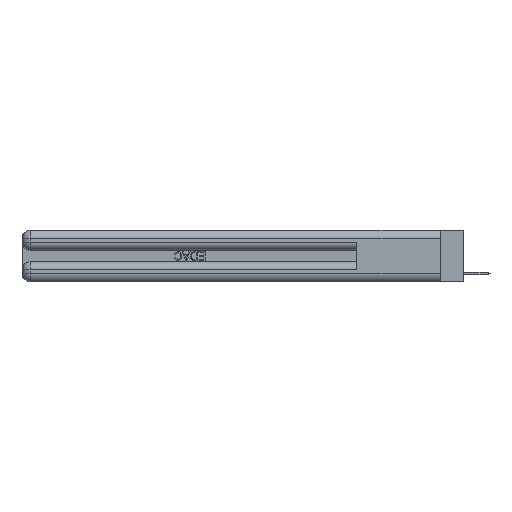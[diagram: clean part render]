
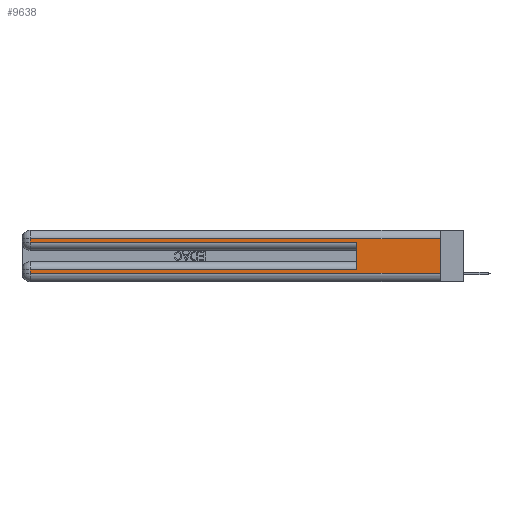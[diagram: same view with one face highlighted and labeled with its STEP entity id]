
A CAD part, left-side view. The second image highlights one B-rep face of the part: STEP entity #9638.
In plain terms, the highlighted planar face has unit normal (-1, 0, 0).
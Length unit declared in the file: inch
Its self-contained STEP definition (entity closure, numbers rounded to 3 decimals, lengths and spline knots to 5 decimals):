
#283 = EDGE_CURVE ( 'NONE', #21786, #4087, #32095, .T. ) ;
#526 = VERTEX_POINT ( 'NONE', #28836 ) ;
#703 = DIRECTION ( 'NONE',  ( 0., 0., 1. ) ) ;
#1009 = VECTOR ( 'NONE', #2353, 39.37008 ) ;
#1032 = VECTOR ( 'NONE', #703, 39.37008 ) ;
#1614 = DIRECTION ( 'NONE',  ( 0., 1., 0. ) ) ;
#2201 = VECTOR ( 'NONE', #23925, 39.37008 ) ;
#2353 = DIRECTION ( 'NONE',  ( 0., -1., 0. ) ) ;
#2397 = LINE ( 'NONE', #23777, #5721 ) ;
#2534 = CARTESIAN_POINT ( 'NONE',  ( 0., 0., 0.37 ) ) ;
#2659 = VERTEX_POINT ( 'NONE', #22991 ) ;
#3039 = LINE ( 'NONE', #2534, #2201 ) ;
#3150 = CARTESIAN_POINT ( 'NONE',  ( 0., 2.94, 0.285 ) ) ;
#4087 = VERTEX_POINT ( 'NONE', #3150 ) ;
#4291 = VERTEX_POINT ( 'NONE', #32530 ) ;
#4304 = ORIENTED_EDGE ( 'NONE', *, *, #19961, .T. ) ;
#4744 = CARTESIAN_POINT ( 'NONE',  ( 0., 2.94, 0.085 ) ) ;
#4871 = AXIS2_PLACEMENT_3D ( 'NONE', #23718, #7321, #32300 ) ;
#5490 = DIRECTION ( 'NONE',  ( 0., 0., -1. ) ) ;
#5721 = VECTOR ( 'NONE', #16513, 39.37008 ) ;
#5727 = CARTESIAN_POINT ( 'NONE',  ( 0., 0., 0.06 ) ) ;
#7321 = DIRECTION ( 'NONE',  ( 1., 0., 0. ) ) ;
#7657 = PLANE ( 'NONE',  #4871 ) ;
#8184 = ORIENTED_EDGE ( 'NONE', *, *, #23989, .T. ) ;
#8616 = VERTEX_POINT ( 'NONE', #9148 ) ;
#8648 = LINE ( 'NONE', #11803, #11957 ) ;
#9148 = CARTESIAN_POINT ( 'NONE',  ( 0., 2.94, 0.06 ) ) ;
#9638 = ADVANCED_FACE ( 'NONE', ( #27715 ), #7657, .F. ) ;
#9937 = LINE ( 'NONE', #5727, #32392 ) ;
#10310 = DIRECTION ( 'NONE',  ( 0., 0., -1. ) ) ;
#11803 = CARTESIAN_POINT ( 'NONE',  ( 0., 0., 0.31 ) ) ;
#11926 = EDGE_CURVE ( 'NONE', #4087, #526, #13859, .T. ) ;
#11957 = VECTOR ( 'NONE', #1614, 39.37008 ) ;
#12534 = VERTEX_POINT ( 'NONE', #4744 ) ;
#12583 = EDGE_CURVE ( 'NONE', #14246, #4291, #3039, .T. ) ;
#13859 = LINE ( 'NONE', #26161, #1009 ) ;
#14246 = VERTEX_POINT ( 'NONE', #32501 ) ;
#15388 = ORIENTED_EDGE ( 'NONE', *, *, #19646, .T. ) ;
#16513 = DIRECTION ( 'NONE',  ( 0., 1., 0. ) ) ;
#17009 = CARTESIAN_POINT ( 'NONE',  ( 0., 0.6, 0.145 ) ) ;
#18685 = CARTESIAN_POINT ( 'NONE',  ( 0., 2.94, 0.37 ) ) ;
#18804 = DIRECTION ( 'NONE',  ( 0., -1., 0. ) ) ;
#19025 = LINE ( 'NONE', #28813, #32328 ) ;
#19646 = EDGE_CURVE ( 'NONE', #14246, #21786, #8648, .T. ) ;
#19961 = EDGE_CURVE ( 'NONE', #2659, #12534, #2397, .T. ) ;
#21786 = VERTEX_POINT ( 'NONE', #27960 ) ;
#22744 = EDGE_LOOP ( 'NONE', ( #26231, #15388, #26869, #31993, #29134, #4304, #8184, #32651 ) ) ;
#22991 = CARTESIAN_POINT ( 'NONE',  ( 0., 0.6, 0.085 ) ) ;
#23718 = CARTESIAN_POINT ( 'NONE',  ( 0., 0., 0.37 ) ) ;
#23777 = CARTESIAN_POINT ( 'NONE',  ( 0., 0., 0.085 ) ) ;
#23925 = DIRECTION ( 'NONE',  ( 0., 0., -1. ) ) ;
#23989 = EDGE_CURVE ( 'NONE', #12534, #8616, #19025, .T. ) ;
#24807 = EDGE_CURVE ( 'NONE', #2659, #526, #32195, .T. ) ;
#26161 = CARTESIAN_POINT ( 'NONE',  ( 0., 0., 0.285 ) ) ;
#26231 = ORIENTED_EDGE ( 'NONE', *, *, #12583, .F. ) ;
#26869 = ORIENTED_EDGE ( 'NONE', *, *, #283, .T. ) ;
#27715 = FACE_OUTER_BOUND ( 'NONE', #22744, .T. ) ;
#27960 = CARTESIAN_POINT ( 'NONE',  ( 0., 2.94, 0.31 ) ) ;
#28813 = CARTESIAN_POINT ( 'NONE',  ( 0., 2.94, 0.37 ) ) ;
#28836 = CARTESIAN_POINT ( 'NONE',  ( 0., 0.6, 0.285 ) ) ;
#29134 = ORIENTED_EDGE ( 'NONE', *, *, #24807, .F. ) ;
#29603 = VECTOR ( 'NONE', #5490, 39.37008 ) ;
#31993 = ORIENTED_EDGE ( 'NONE', *, *, #11926, .T. ) ;
#32095 = LINE ( 'NONE', #18685, #29603 ) ;
#32195 = LINE ( 'NONE', #17009, #1032 ) ;
#32300 = DIRECTION ( 'NONE',  ( 0., 0., -1. ) ) ;
#32328 = VECTOR ( 'NONE', #10310, 39.37008 ) ;
#32392 = VECTOR ( 'NONE', #18804, 39.37008 ) ;
#32501 = CARTESIAN_POINT ( 'NONE',  ( 0., 0., 0.31 ) ) ;
#32530 = CARTESIAN_POINT ( 'NONE',  ( 0., 0., 0.06 ) ) ;
#32651 = ORIENTED_EDGE ( 'NONE', *, *, #32768, .T. ) ;
#32768 = EDGE_CURVE ( 'NONE', #8616, #4291, #9937, .T. ) ;
